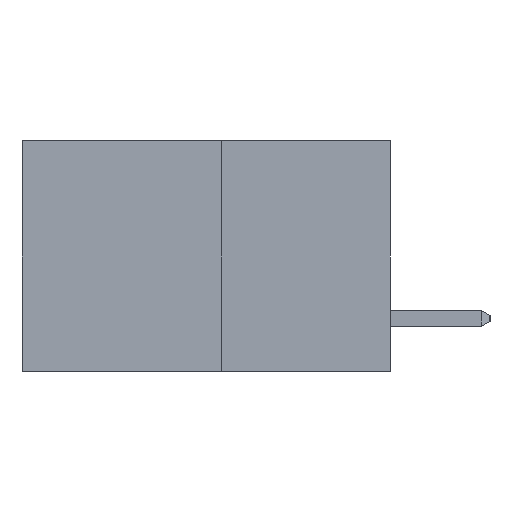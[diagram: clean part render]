
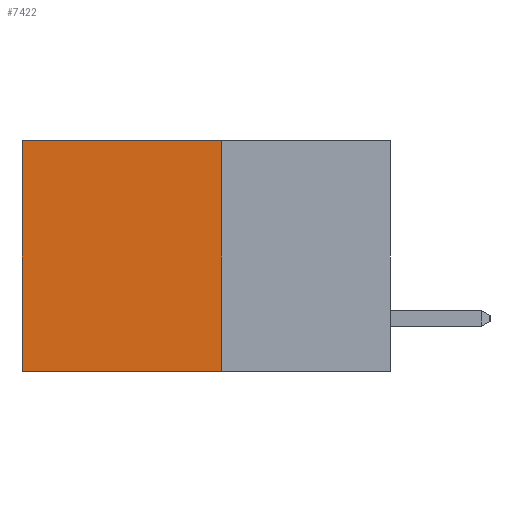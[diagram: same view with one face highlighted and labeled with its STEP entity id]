
A CAD part, left-side view. The second image highlights one B-rep face of the part: STEP entity #7422.
In plain terms, the highlighted planar face has unit normal (-1, 0, 0).
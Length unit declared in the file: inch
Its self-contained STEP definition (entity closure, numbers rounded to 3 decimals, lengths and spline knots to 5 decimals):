
#503 = ORIENTED_EDGE ( 'NONE', *, *, #9669, .F. ) ;
#1088 = LINE ( 'NONE', #6136, #3826 ) ;
#1492 = LINE ( 'NONE', #5007, #12736 ) ;
#1562 = VERTEX_POINT ( 'NONE', #2698 ) ;
#1637 = DIRECTION ( 'NONE',  ( 0., 0., -1. ) ) ;
#2156 = LINE ( 'NONE', #4684, #8440 ) ;
#2698 = CARTESIAN_POINT ( 'NONE',  ( 0.277, 0.59, 0. ) ) ;
#2751 = ORIENTED_EDGE ( 'NONE', *, *, #12735, .F. ) ;
#3360 = CARTESIAN_POINT ( 'NONE',  ( 0.277, 0.27, 0. ) ) ;
#3826 = VECTOR ( 'NONE', #10371, 39.37008 ) ;
#3850 = CARTESIAN_POINT ( 'NONE',  ( 0.277, 0.27, 0. ) ) ;
#4684 = CARTESIAN_POINT ( 'NONE',  ( 0.277, 0.27, -0.37 ) ) ;
#5007 = CARTESIAN_POINT ( 'NONE',  ( 0.277, 0.27, -0.37 ) ) ;
#6136 = CARTESIAN_POINT ( 'NONE',  ( 0.277, 0.59, -0.37 ) ) ;
#6251 = CARTESIAN_POINT ( 'NONE',  ( 0.277, 0.59, -0.37 ) ) ;
#6978 = DIRECTION ( 'NONE',  ( 0., 1., 0. ) ) ;
#7074 = LINE ( 'NONE', #3360, #12008 ) ;
#7422 = ADVANCED_FACE ( 'NONE', ( #14116 ), #10297, .F. ) ;
#8440 = VECTOR ( 'NONE', #6978, 39.37008 ) ;
#9669 = EDGE_CURVE ( 'NONE', #13498, #13958, #1492, .T. ) ;
#9722 = VERTEX_POINT ( 'NONE', #6251 ) ;
#9733 = DIRECTION ( 'NONE',  ( 0., 0., -1. ) ) ;
#9883 = DIRECTION ( 'NONE',  ( 0., 1., 0. ) ) ;
#10110 = DIRECTION ( 'NONE',  ( 1., 0., 0. ) ) ;
#10297 = PLANE ( 'NONE',  #13491 ) ;
#10371 = DIRECTION ( 'NONE',  ( 0., 0., -1. ) ) ;
#11064 = CARTESIAN_POINT ( 'NONE',  ( 0.277, 0.27, -0.37 ) ) ;
#11725 = CARTESIAN_POINT ( 'NONE',  ( 0.277, 0.27, -0.37 ) ) ;
#12008 = VECTOR ( 'NONE', #9883, 39.37008 ) ;
#12012 = EDGE_CURVE ( 'NONE', #1562, #9722, #1088, .T. ) ;
#12735 = EDGE_CURVE ( 'NONE', #13958, #9722, #2156, .T. ) ;
#12736 = VECTOR ( 'NONE', #1637, 39.37008 ) ;
#13073 = ORIENTED_EDGE ( 'NONE', *, *, #13229, .T. ) ;
#13229 = EDGE_CURVE ( 'NONE', #13498, #1562, #7074, .T. ) ;
#13491 = AXIS2_PLACEMENT_3D ( 'NONE', #11725, #10110, #9733 ) ;
#13498 = VERTEX_POINT ( 'NONE', #3850 ) ;
#13527 = EDGE_LOOP ( 'NONE', ( #13709, #2751, #503, #13073 ) ) ;
#13709 = ORIENTED_EDGE ( 'NONE', *, *, #12012, .T. ) ;
#13958 = VERTEX_POINT ( 'NONE', #11064 ) ;
#14116 = FACE_OUTER_BOUND ( 'NONE', #13527, .T. ) ;
